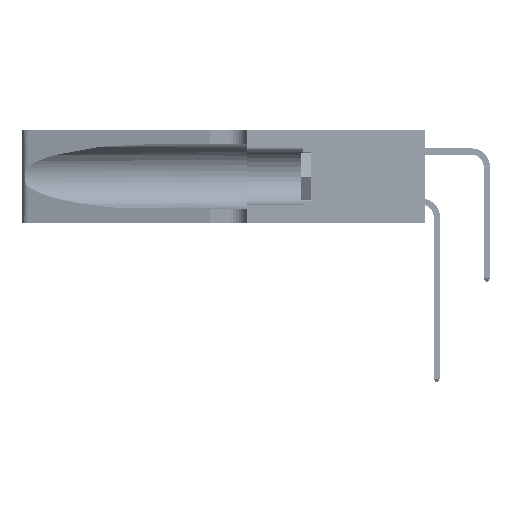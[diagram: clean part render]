
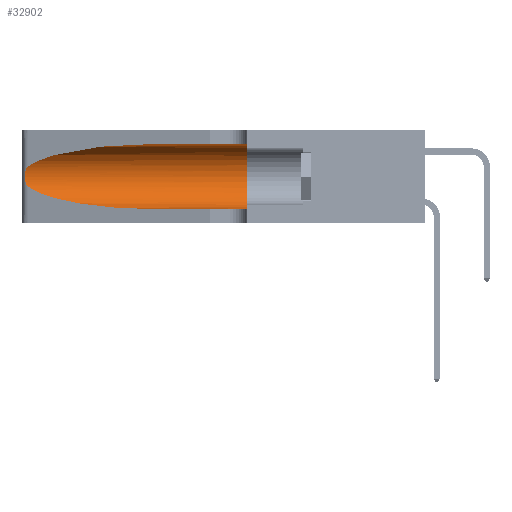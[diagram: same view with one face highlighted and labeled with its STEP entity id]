
A CAD part, left-side view. The second image highlights one B-rep face of the part: STEP entity #32902.
In plain terms, the highlighted cylindrical face has radius 3.308 mm (diameter 6.617 mm), a partial arc.
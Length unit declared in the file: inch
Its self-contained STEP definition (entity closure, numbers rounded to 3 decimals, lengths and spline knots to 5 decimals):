
#1258 = CARTESIAN_POINT ( 'NONE',  ( 0.18966, 0.96281, 0.05475 ) ) ;
#1958 = CYLINDRICAL_SURFACE ( 'NONE', #4130, 0.13025 ) ;
#3481 = ORIENTED_EDGE ( 'NONE', *, *, #35227, .T. ) ;
#3486 = CARTESIAN_POINT ( 'NONE',  ( 0.25854, 1.2359, 0.20912 ) ) ;
#3980 = CARTESIAN_POINT ( 'NONE',  ( 0.2373, 1.15595, 0.28018 ) ) ;
#4130 = AXIS2_PLACEMENT_3D ( 'NONE', #54018, #49715, #28332 ) ;
#5269 = CARTESIAN_POINT ( 'NONE',  ( 0.25487, 1.22718, 0.14631 ) ) ;
#6145 = LINE ( 'NONE', #13863, #16313 ) ;
#6700 = ORIENTED_EDGE ( 'NONE', *, *, #33331, .T. ) ;
#7100 = EDGE_CURVE ( 'NONE', #19359, #46362, #18461, .T. ) ;
#7351 = CARTESIAN_POINT ( 'NONE',  ( 0.1305, 0.35, 0.31525 ) ) ;
#7878 = CARTESIAN_POINT ( 'NONE',  ( 0.26075, 1.23896, 0.19203 ) ) ;
#10302 = VECTOR ( 'NONE', #45156, 39.37008 ) ;
#10550 = EDGE_LOOP ( 'NONE', ( #14295, #19003, #6700, #3481, #38475, #29336 ) ) ;
#12239 = CARTESIAN_POINT ( 'NONE',  ( 0.26017, 1.23833, 0.17102 ) ) ;
#12592 = EDGE_CURVE ( 'NONE', #16741, #32988, #39093, .T. ) ;
#13863 = CARTESIAN_POINT ( 'NONE',  ( 0.1305, 1.61858, 0.05475 ) ) ;
#14148 = CARTESIAN_POINT ( 'NONE',  ( 0.2373, 1.15595, 0.08982 ) ) ;
#14295 = ORIENTED_EDGE ( 'NONE', *, *, #7100, .T. ) ;
#14938 = DIRECTION ( 'NONE',  ( 0., 1., 0. ) ) ;
#16218 = FACE_OUTER_BOUND ( 'NONE', #10550, .T. ) ;
#16313 = VECTOR ( 'NONE', #31609, 39.37008 ) ;
#16400 = CARTESIAN_POINT ( 'NONE',  ( 0.25555, 1.22994, 0.2215 ) ) ;
#16599 = CARTESIAN_POINT ( 'NONE',  ( 0.25789, 1.23486, 0.15765 ) ) ;
#16741 = VERTEX_POINT ( 'NONE', #7351 ) ;
#18461 =( BOUNDED_CURVE ( )  B_SPLINE_CURVE ( 3, ( #29862, #34217, #3980, #38532 ),
 .UNSPECIFIED., .F., .F. ) 
 B_SPLINE_CURVE_WITH_KNOTS ( ( 4, 4 ),
 ( 1.5708, 2.84003 ),
 .UNSPECIFIED. ) 
 CURVE ( )  GEOMETRIC_REPRESENTATION_ITEM ( )  RATIONAL_B_SPLINE_CURVE ( ( 1., 0.87, 0.87, 1. ) ) 
 REPRESENTATION_ITEM ( '' )  );
#18516 = CARTESIAN_POINT ( 'NONE',  ( 0.25487, 1.22718, 0.14631 ) ) ;
#19003 = ORIENTED_EDGE ( 'NONE', *, *, #33661, .T. ) ;
#19359 = VERTEX_POINT ( 'NONE', #51050 ) ;
#19419 = CARTESIAN_POINT ( 'NONE',  ( 0.1305, 1.61858, 0.31525 ) ) ;
#20419 = CARTESIAN_POINT ( 'NONE',  ( 0.1305, 0.35, 0.05475 ) ) ;
#20912 = CARTESIAN_POINT ( 'NONE',  ( 0.25555, 1.22993, 0.14849 ) ) ;
#21743 = LINE ( 'NONE', #19419, #10302 ) ;
#28332 = DIRECTION ( 'NONE',  ( 0., 0., -1. ) ) ;
#29336 = ORIENTED_EDGE ( 'NONE', *, *, #30716, .F. ) ;
#29382 = CARTESIAN_POINT ( 'NONE',  ( 0.25787, 1.23484, 0.2124 ) ) ;
#29862 = CARTESIAN_POINT ( 'NONE',  ( 0.1305, 0.72297, 0.31525 ) ) ;
#30268 = CARTESIAN_POINT ( 'NONE',  ( 0.25487, 1.22718, 0.22369 ) ) ;
#30716 = EDGE_CURVE ( 'NONE', #19359, #16741, #21743, .T. ) ;
#31399 = VERTEX_POINT ( 'NONE', #5269 ) ;
#31526 = CARTESIAN_POINT ( 'NONE',  ( 0.1305, 0.72297, 0.05475 ) ) ;
#31609 = DIRECTION ( 'NONE',  ( 0., -1., 0. ) ) ;
#32902 = ADVANCED_FACE ( 'NONE', ( #16218 ), #1958, .F. ) ;
#32988 = VERTEX_POINT ( 'NONE', #20419 ) ;
#33331 = EDGE_CURVE ( 'NONE', #31399, #37891, #50117, .T. ) ;
#33661 = EDGE_CURVE ( 'NONE', #46362, #31399, #40173, .T. ) ;
#33720 = CARTESIAN_POINT ( 'NONE',  ( 0.26018, 1.23835, 0.19895 ) ) ;
#33918 = AXIS2_PLACEMENT_3D ( 'NONE', #40732, #14938, #45036 ) ;
#34217 = CARTESIAN_POINT ( 'NONE',  ( 0.18966, 0.96281, 0.31525 ) ) ;
#35227 = EDGE_CURVE ( 'NONE', #37891, #32988, #6145, .T. ) ;
#37891 = VERTEX_POINT ( 'NONE', #50146 ) ;
#38046 = CARTESIAN_POINT ( 'NONE',  ( 0.26075, 1.23896, 0.178 ) ) ;
#38475 = ORIENTED_EDGE ( 'NONE', *, *, #12592, .F. ) ;
#38532 = CARTESIAN_POINT ( 'NONE',  ( 0.25487, 1.22718, 0.22369 ) ) ;
#39093 = CIRCLE ( 'NONE', #33918, 0.13025 ) ;
#40173 = B_SPLINE_CURVE_WITH_KNOTS ( 'NONE', 3,
 ( #42162, #16400, #55071, #29382, #3486, #33720, #7878, #38046, #12239, #42344, #16599, #46639, #20912, #50948 ),
 .UNSPECIFIED., .F., .F.,
 ( 4, 2, 2, 2, 2, 2, 4 ),
 ( 0., 0.00027, 0.00053, 0.00107, 0.0016, 0.00187, 0.00214 ),
 .UNSPECIFIED. ) ;
#40732 = CARTESIAN_POINT ( 'NONE',  ( 0.1305, 0.35, 0.185 ) ) ;
#42162 = CARTESIAN_POINT ( 'NONE',  ( 0.25487, 1.22718, 0.22369 ) ) ;
#42344 = CARTESIAN_POINT ( 'NONE',  ( 0.25856, 1.23593, 0.16098 ) ) ;
#45036 = DIRECTION ( 'NONE',  ( 0., 0., 1. ) ) ;
#45156 = DIRECTION ( 'NONE',  ( 0., -1., 0. ) ) ;
#46362 = VERTEX_POINT ( 'NONE', #30268 ) ;
#46639 = CARTESIAN_POINT ( 'NONE',  ( 0.25639, 1.23186, 0.15144 ) ) ;
#49715 = DIRECTION ( 'NONE',  ( 0., -1., 0. ) ) ;
#50117 =( BOUNDED_CURVE ( )  B_SPLINE_CURVE ( 3, ( #18516, #14148, #1258, #31526 ),
 .UNSPECIFIED., .F., .F. ) 
 B_SPLINE_CURVE_WITH_KNOTS ( ( 4, 4 ),
 ( 3.44316, 4.71239 ),
 .UNSPECIFIED. ) 
 CURVE ( )  GEOMETRIC_REPRESENTATION_ITEM ( )  RATIONAL_B_SPLINE_CURVE ( ( 1., 0.87, 0.87, 1. ) ) 
 REPRESENTATION_ITEM ( '' )  );
#50146 = CARTESIAN_POINT ( 'NONE',  ( 0.1305, 0.72297, 0.05475 ) ) ;
#50948 = CARTESIAN_POINT ( 'NONE',  ( 0.25487, 1.22718, 0.14631 ) ) ;
#51050 = CARTESIAN_POINT ( 'NONE',  ( 0.1305, 0.72297, 0.31525 ) ) ;
#54018 = CARTESIAN_POINT ( 'NONE',  ( 0.1305, 1.61858, 0.185 ) ) ;
#55071 = CARTESIAN_POINT ( 'NONE',  ( 0.25639, 1.23184, 0.21858 ) ) ;
